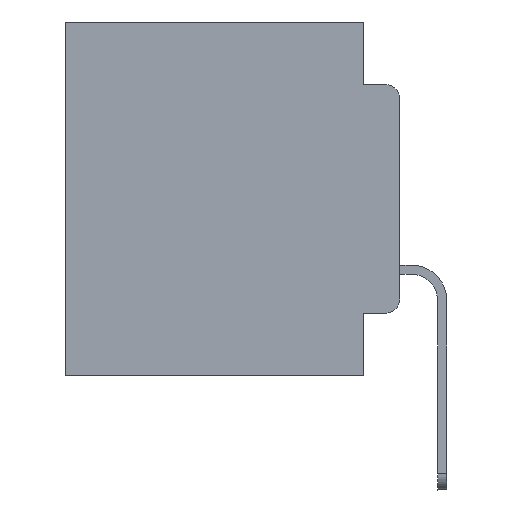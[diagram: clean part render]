
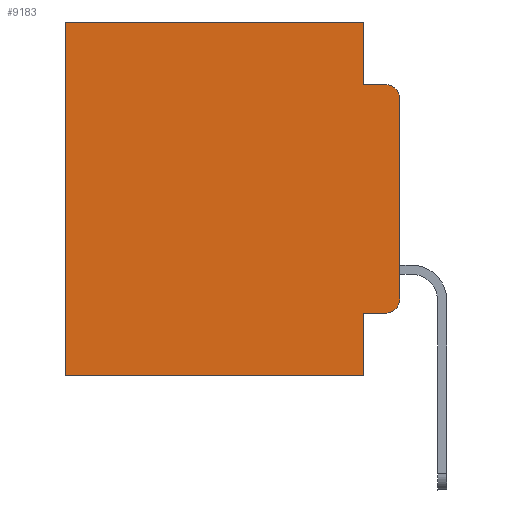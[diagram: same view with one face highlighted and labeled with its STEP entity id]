
A CAD part, left-side view. The second image highlights one B-rep face of the part: STEP entity #9183.
In plain terms, the highlighted planar face has unit normal (-1, 0, 0).
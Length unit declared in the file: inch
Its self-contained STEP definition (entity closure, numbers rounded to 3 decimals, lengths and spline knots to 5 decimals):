
#161 = LINE ( 'NONE', #15958, #7494 ) ;
#518 = CARTESIAN_POINT ( 'NONE',  ( 0.298, 0.02, -0.1085 ) ) ;
#595 = DIRECTION ( 'NONE',  ( 0., 0., -1. ) ) ;
#964 = CARTESIAN_POINT ( 'NONE',  ( 0.298, 0., 0. ) ) ;
#1104 = CARTESIAN_POINT ( 'NONE',  ( 0.298, 0., -0.3915 ) ) ;
#1355 = PLANE ( 'NONE',  #3468 ) ;
#1368 = CARTESIAN_POINT ( 'NONE',  ( 0.298, 0.473, 0. ) ) ;
#1857 = CARTESIAN_POINT ( 'NONE',  ( 0.298, 0.051, -0.5 ) ) ;
#1935 = EDGE_CURVE ( 'NONE', #4939, #2359, #21868, .T. ) ;
#2359 = VERTEX_POINT ( 'NONE', #25217 ) ;
#2779 = DIRECTION ( 'NONE',  ( -1., 0., 0. ) ) ;
#2816 = CARTESIAN_POINT ( 'NONE',  ( 0.298, 0.051, 0. ) ) ;
#3468 = AXIS2_PLACEMENT_3D ( 'NONE', #964, #5089, #15041 ) ;
#3923 = CARTESIAN_POINT ( 'NONE',  ( 0.298, 0.051, 0. ) ) ;
#4187 = LINE ( 'NONE', #6952, #4561 ) ;
#4561 = VECTOR ( 'NONE', #15030, 39.37008 ) ;
#4742 = DIRECTION ( 'NONE',  ( 0., 0., -1. ) ) ;
#4939 = VERTEX_POINT ( 'NONE', #19374 ) ;
#4940 = CARTESIAN_POINT ( 'NONE',  ( 0.298, 0.02, -0.4115 ) ) ;
#5089 = DIRECTION ( 'NONE',  ( 1., 0., 0. ) ) ;
#5791 = VERTEX_POINT ( 'NONE', #1104 ) ;
#6079 = VECTOR ( 'NONE', #19546, 39.37008 ) ;
#6142 = VERTEX_POINT ( 'NONE', #21635 ) ;
#6952 = CARTESIAN_POINT ( 'NONE',  ( 0.298, 0.051, 0. ) ) ;
#7494 = VECTOR ( 'NONE', #24228, 39.37008 ) ;
#8036 = CARTESIAN_POINT ( 'NONE',  ( 0.298, 0.473, -0.5 ) ) ;
#9077 = ORIENTED_EDGE ( 'NONE', *, *, #18011, .T. ) ;
#9183 = ADVANCED_FACE ( 'NONE', ( #11449 ), #1355, .F. ) ;
#9320 = LINE ( 'NONE', #17419, #20339 ) ;
#9513 = LINE ( 'NONE', #17610, #13922 ) ;
#9685 = CARTESIAN_POINT ( 'NONE',  ( 0.298, 0., 0. ) ) ;
#10408 = AXIS2_PLACEMENT_3D ( 'NONE', #518, #2779, #19128 ) ;
#10688 = CARTESIAN_POINT ( 'NONE',  ( 0.298, 0.051, -0.4115 ) ) ;
#10832 = CARTESIAN_POINT ( 'NONE',  ( 0.298, 0.473, 0. ) ) ;
#10939 = VECTOR ( 'NONE', #595, 39.37008 ) ;
#11431 = LINE ( 'NONE', #13670, #6079 ) ;
#11449 = FACE_OUTER_BOUND ( 'NONE', #25988, .T. ) ;
#11540 = VERTEX_POINT ( 'NONE', #8036 ) ;
#11565 = VERTEX_POINT ( 'NONE', #10688 ) ;
#11769 = LINE ( 'NONE', #3923, #12190 ) ;
#11799 = ORIENTED_EDGE ( 'NONE', *, *, #24561, .F. ) ;
#11966 = ORIENTED_EDGE ( 'NONE', *, *, #1935, .T. ) ;
#12021 = DIRECTION ( 'NONE',  ( 0., 0., -1. ) ) ;
#12190 = VECTOR ( 'NONE', #12021, 39.37008 ) ;
#12263 = EDGE_CURVE ( 'NONE', #16534, #11540, #11431, .T. ) ;
#12931 = CIRCLE ( 'NONE', #16306, 0.02 ) ;
#13406 = DIRECTION ( 'NONE',  ( 0., 1., 0. ) ) ;
#13519 = LINE ( 'NONE', #9685, #18251 ) ;
#13670 = CARTESIAN_POINT ( 'NONE',  ( 0.298, 0., -0.5 ) ) ;
#13922 = VECTOR ( 'NONE', #25735, 39.37008 ) ;
#14678 = ORIENTED_EDGE ( 'NONE', *, *, #23132, .F. ) ;
#14925 = LINE ( 'NONE', #10832, #10939 ) ;
#15030 = DIRECTION ( 'NONE',  ( 0., 0., -1. ) ) ;
#15041 = DIRECTION ( 'NONE',  ( 0., 0., -1. ) ) ;
#15544 = EDGE_CURVE ( 'NONE', #11565, #25762, #9513, .T. ) ;
#15614 = ORIENTED_EDGE ( 'NONE', *, *, #15544, .T. ) ;
#15958 = CARTESIAN_POINT ( 'NONE',  ( 0.298, 0.051, -0.0885 ) ) ;
#16306 = AXIS2_PLACEMENT_3D ( 'NONE', #22959, #21343, #4742 ) ;
#16534 = VERTEX_POINT ( 'NONE', #1857 ) ;
#16873 = ORIENTED_EDGE ( 'NONE', *, *, #24395, .F. ) ;
#17419 = CARTESIAN_POINT ( 'NONE',  ( 0.298, 0., 0. ) ) ;
#17610 = CARTESIAN_POINT ( 'NONE',  ( 0.298, 0.051, -0.4115 ) ) ;
#17790 = DIRECTION ( 'NONE',  ( 0., 0., -1. ) ) ;
#18011 = EDGE_CURVE ( 'NONE', #23222, #21685, #9320, .T. ) ;
#18251 = VECTOR ( 'NONE', #17790, 39.37008 ) ;
#18619 = EDGE_CURVE ( 'NONE', #4939, #5791, #13519, .T. ) ;
#19128 = DIRECTION ( 'NONE',  ( 0., 0., -1. ) ) ;
#19374 = CARTESIAN_POINT ( 'NONE',  ( 0.298, 0., -0.1085 ) ) ;
#19546 = DIRECTION ( 'NONE',  ( 0., 1., 0. ) ) ;
#19624 = ORIENTED_EDGE ( 'NONE', *, *, #22765, .T. ) ;
#20136 = EDGE_CURVE ( 'NONE', #25762, #5791, #12931, .T. ) ;
#20339 = VECTOR ( 'NONE', #13406, 39.37008 ) ;
#20394 = ORIENTED_EDGE ( 'NONE', *, *, #18619, .F. ) ;
#21248 = ORIENTED_EDGE ( 'NONE', *, *, #12263, .F. ) ;
#21343 = DIRECTION ( 'NONE',  ( -1., 0., 0. ) ) ;
#21635 = CARTESIAN_POINT ( 'NONE',  ( 0.298, 0.051, -0.0885 ) ) ;
#21685 = VERTEX_POINT ( 'NONE', #1368 ) ;
#21868 = CIRCLE ( 'NONE', #10408, 0.02 ) ;
#22765 = EDGE_CURVE ( 'NONE', #21685, #11540, #14925, .T. ) ;
#22959 = CARTESIAN_POINT ( 'NONE',  ( 0.298, 0.02, -0.3915 ) ) ;
#23132 = EDGE_CURVE ( 'NONE', #6142, #2359, #161, .T. ) ;
#23222 = VERTEX_POINT ( 'NONE', #2816 ) ;
#23819 = ORIENTED_EDGE ( 'NONE', *, *, #20136, .T. ) ;
#24228 = DIRECTION ( 'NONE',  ( 0., -1., 0. ) ) ;
#24395 = EDGE_CURVE ( 'NONE', #23222, #6142, #11769, .T. ) ;
#24561 = EDGE_CURVE ( 'NONE', #11565, #16534, #4187, .T. ) ;
#25217 = CARTESIAN_POINT ( 'NONE',  ( 0.298, 0.02, -0.0885 ) ) ;
#25735 = DIRECTION ( 'NONE',  ( 0., -1., 0. ) ) ;
#25762 = VERTEX_POINT ( 'NONE', #4940 ) ;
#25988 = EDGE_LOOP ( 'NONE', ( #20394, #11966, #14678, #16873, #9077, #19624, #21248, #11799, #15614, #23819 ) ) ;
